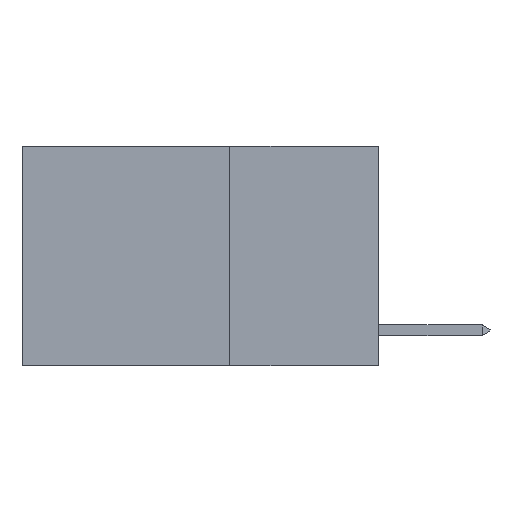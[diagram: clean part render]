
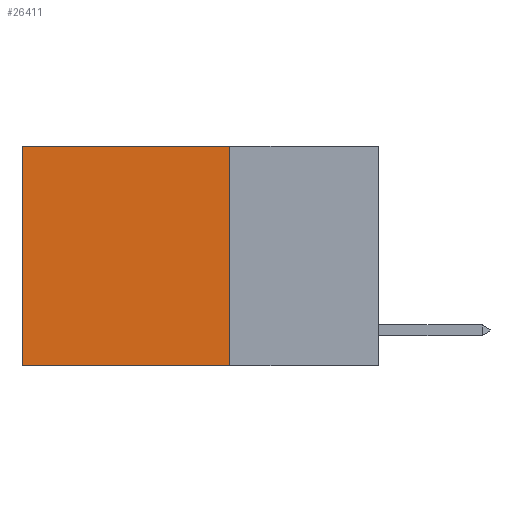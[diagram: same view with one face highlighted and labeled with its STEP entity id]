
A CAD part, left-side view. The second image highlights one B-rep face of the part: STEP entity #26411.
In plain terms, the highlighted planar face has unit normal (-1, 0, 0).
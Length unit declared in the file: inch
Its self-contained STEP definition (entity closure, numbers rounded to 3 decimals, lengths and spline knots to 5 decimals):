
#155 = CARTESIAN_POINT ( 'NONE',  ( 0.2625, 0.25, 0. ) ) ;
#750 = VERTEX_POINT ( 'NONE', #22912 ) ;
#974 = ORIENTED_EDGE ( 'NONE', *, *, #22662, .T. ) ;
#2059 = VERTEX_POINT ( 'NONE', #14582 ) ;
#2083 = DIRECTION ( 'NONE',  ( 0., 0., -1. ) ) ;
#4222 = CARTESIAN_POINT ( 'NONE',  ( 0.2625, 0.25, -0.37 ) ) ;
#6214 = LINE ( 'NONE', #155, #17290 ) ;
#6488 = DIRECTION ( 'NONE',  ( 0., 1., 0. ) ) ;
#6556 = CARTESIAN_POINT ( 'NONE',  ( 0.2625, 0.25, 0. ) ) ;
#6635 = LINE ( 'NONE', #4222, #11892 ) ;
#6740 = VECTOR ( 'NONE', #2083, 39.37008 ) ;
#7520 = EDGE_CURVE ( 'NONE', #28237, #2059, #18486, .T. ) ;
#7959 = LINE ( 'NONE', #21835, #17623 ) ;
#8126 = FACE_OUTER_BOUND ( 'NONE', #20851, .T. ) ;
#9627 = ORIENTED_EDGE ( 'NONE', *, *, #10960, .T. ) ;
#9719 = DIRECTION ( 'NONE',  ( 1., 0., 0. ) ) ;
#10060 = ORIENTED_EDGE ( 'NONE', *, *, #7520, .F. ) ;
#10960 = EDGE_CURVE ( 'NONE', #750, #25900, #7959, .T. ) ;
#11886 = CARTESIAN_POINT ( 'NONE',  ( 0.2625, 0.25, 0. ) ) ;
#11892 = VECTOR ( 'NONE', #6488, 39.37008 ) ;
#13635 = DIRECTION ( 'NONE',  ( 0., 1., 0. ) ) ;
#14582 = CARTESIAN_POINT ( 'NONE',  ( 0.2625, 0.25, -0.37 ) ) ;
#16119 = EDGE_CURVE ( 'NONE', #2059, #25900, #6635, .T. ) ;
#16703 = CARTESIAN_POINT ( 'NONE',  ( 0.2625, 0.6, -0.37 ) ) ;
#17290 = VECTOR ( 'NONE', #13635, 39.37008 ) ;
#17623 = VECTOR ( 'NONE', #24005, 39.37008 ) ;
#18473 = PLANE ( 'NONE',  #23850 ) ;
#18486 = LINE ( 'NONE', #6556, #6740 ) ;
#20851 = EDGE_LOOP ( 'NONE', ( #9627, #24753, #10060, #974 ) ) ;
#21417 = CARTESIAN_POINT ( 'NONE',  ( 0.2625, 0.25, 0. ) ) ;
#21835 = CARTESIAN_POINT ( 'NONE',  ( 0.2625, 0.6, 0. ) ) ;
#22662 = EDGE_CURVE ( 'NONE', #28237, #750, #6214, .T. ) ;
#22912 = CARTESIAN_POINT ( 'NONE',  ( 0.2625, 0.6, 0. ) ) ;
#23850 = AXIS2_PLACEMENT_3D ( 'NONE', #11886, #9719, #25024 ) ;
#24005 = DIRECTION ( 'NONE',  ( 0., 0., -1. ) ) ;
#24753 = ORIENTED_EDGE ( 'NONE', *, *, #16119, .F. ) ;
#25024 = DIRECTION ( 'NONE',  ( 0., 0., -1. ) ) ;
#25900 = VERTEX_POINT ( 'NONE', #16703 ) ;
#26411 = ADVANCED_FACE ( 'NONE', ( #8126 ), #18473, .F. ) ;
#28237 = VERTEX_POINT ( 'NONE', #21417 ) ;
